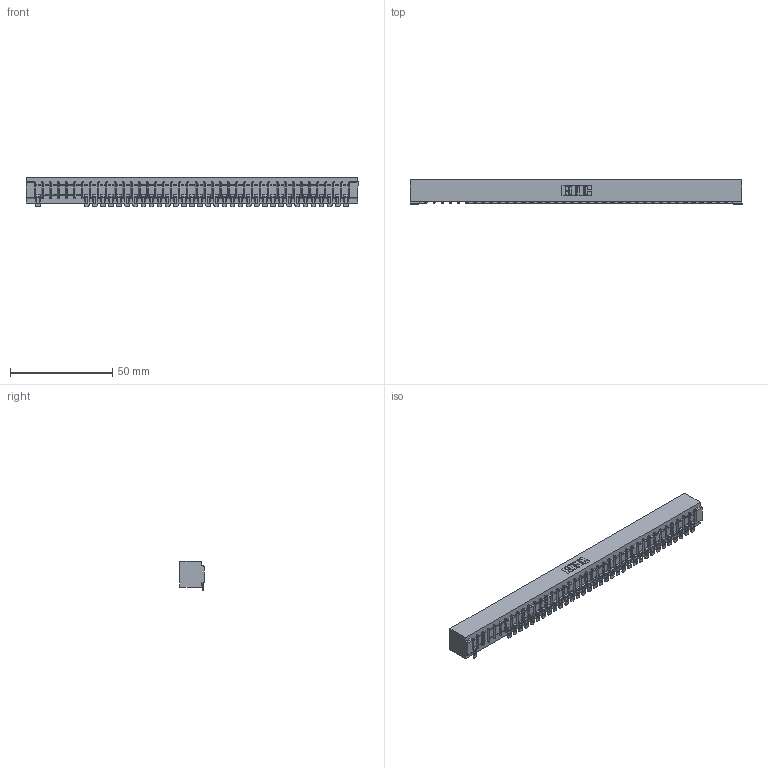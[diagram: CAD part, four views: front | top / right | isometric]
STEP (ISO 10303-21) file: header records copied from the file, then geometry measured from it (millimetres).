
FILE_DESCRIPTION (( 'STEP AP203' ), '1' );
FILE_NAME ('357-039-554-101.STEP', '2018-08-11T04:27:57', ( '' ), ( '' ), 'SwSTEP 2.0', 'SolidWorks 2016', '' );
FILE_SCHEMA (( 'CONFIG_CONTROL_DESIGN' ));
Length unit declared in the file: inch
Products named in the file (3): 307 Part_No Mounting Lugs; 307-290-002_554; 357-039-554-101
Assembly tree (35 placements, depth 2):
  357-039-554-101
    307 Part_No Mounting Lugs
    307-290-002_554  x34
Bounding box: 162.41 x 12.01 x 14.52 mm (x, y, z)
Volume: 17782.6 mm3; surface area: 21847.2 mm2
Topology: 35 solids, 35 shells, 3004 faces, 9221 edges, 6038 vertices
Faces by surface type: plane 1690, cylinder 1234, sphere 80
Entity records: 34331 total; most frequent: CARTESIAN_POINT 5813, ORIENTED_EDGE 5808, DIRECTION 5648, EDGE_CURVE 2904, VECTOR 2218, LINE 2218, VERTEX_POINT 1880, AXIS2_PLACEMENT_3D 1715
